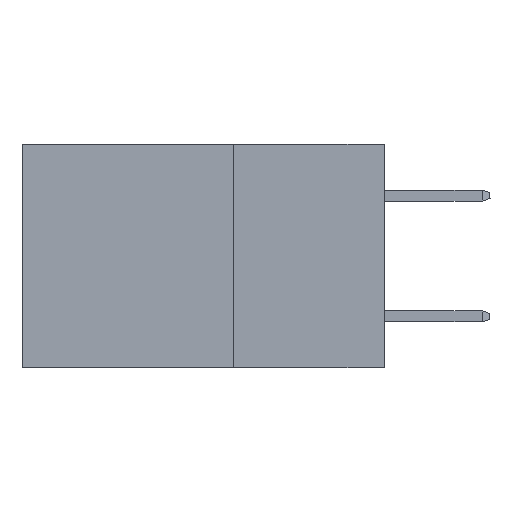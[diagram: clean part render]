
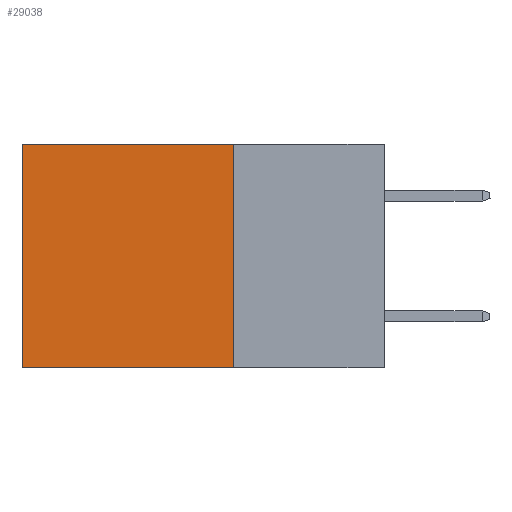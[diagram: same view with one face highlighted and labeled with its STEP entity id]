
A CAD part, left-side view. The second image highlights one B-rep face of the part: STEP entity #29038.
In plain terms, the highlighted planar face has unit normal (-1, 0, 0).
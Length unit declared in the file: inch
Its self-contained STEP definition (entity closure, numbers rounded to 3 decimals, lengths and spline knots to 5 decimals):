
#643 = DIRECTION ( 'NONE',  ( 0., 1., 0. ) ) ;
#678 = CARTESIAN_POINT ( 'NONE',  ( 0.298, 0.25, 0. ) ) ;
#2211 = CARTESIAN_POINT ( 'NONE',  ( 0.298, 0.25, 0. ) ) ;
#2407 = VERTEX_POINT ( 'NONE', #11066 ) ;
#2975 = DIRECTION ( 'NONE',  ( 0., 0., -1. ) ) ;
#3586 = CARTESIAN_POINT ( 'NONE',  ( 0.298, 0.25, 0. ) ) ;
#4571 = EDGE_CURVE ( 'NONE', #28211, #2407, #26908, .T. ) ;
#5123 = AXIS2_PLACEMENT_3D ( 'NONE', #3586, #24523, #10641 ) ;
#7602 = CARTESIAN_POINT ( 'NONE',  ( 0.298, 0.25, 0. ) ) ;
#7730 = VECTOR ( 'NONE', #9236, 39.37008 ) ;
#9236 = DIRECTION ( 'NONE',  ( 0., 0., -1. ) ) ;
#9410 = VERTEX_POINT ( 'NONE', #24506 ) ;
#9896 = ORIENTED_EDGE ( 'NONE', *, *, #16521, .T. ) ;
#10234 = EDGE_CURVE ( 'NONE', #2407, #9410, #22271, .T. ) ;
#10473 = LINE ( 'NONE', #28382, #21373 ) ;
#10641 = DIRECTION ( 'NONE',  ( 0., 0., -1. ) ) ;
#10811 = CARTESIAN_POINT ( 'NONE',  ( 0.298, 0.6, 0. ) ) ;
#11066 = CARTESIAN_POINT ( 'NONE',  ( 0.298, 0.25, -0.37 ) ) ;
#12013 = FACE_OUTER_BOUND ( 'NONE', #17609, .T. ) ;
#15255 = PLANE ( 'NONE',  #5123 ) ;
#16161 = VECTOR ( 'NONE', #27747, 39.37008 ) ;
#16521 = EDGE_CURVE ( 'NONE', #27720, #9410, #10473, .T. ) ;
#16907 = LINE ( 'NONE', #7602, #21570 ) ;
#17609 = EDGE_LOOP ( 'NONE', ( #9896, #17995, #27429, #28494 ) ) ;
#17995 = ORIENTED_EDGE ( 'NONE', *, *, #10234, .F. ) ;
#21373 = VECTOR ( 'NONE', #2975, 39.37008 ) ;
#21570 = VECTOR ( 'NONE', #643, 39.37008 ) ;
#22271 = LINE ( 'NONE', #25367, #16161 ) ;
#24506 = CARTESIAN_POINT ( 'NONE',  ( 0.298, 0.6, -0.37 ) ) ;
#24523 = DIRECTION ( 'NONE',  ( 1., 0., 0. ) ) ;
#25367 = CARTESIAN_POINT ( 'NONE',  ( 0.298, 0.25, -0.37 ) ) ;
#26750 = EDGE_CURVE ( 'NONE', #28211, #27720, #16907, .T. ) ;
#26908 = LINE ( 'NONE', #2211, #7730 ) ;
#27429 = ORIENTED_EDGE ( 'NONE', *, *, #4571, .F. ) ;
#27720 = VERTEX_POINT ( 'NONE', #10811 ) ;
#27747 = DIRECTION ( 'NONE',  ( 0., 1., 0. ) ) ;
#28211 = VERTEX_POINT ( 'NONE', #678 ) ;
#28382 = CARTESIAN_POINT ( 'NONE',  ( 0.298, 0.6, 0. ) ) ;
#28494 = ORIENTED_EDGE ( 'NONE', *, *, #26750, .T. ) ;
#29038 = ADVANCED_FACE ( 'NONE', ( #12013 ), #15255, .F. ) ;
